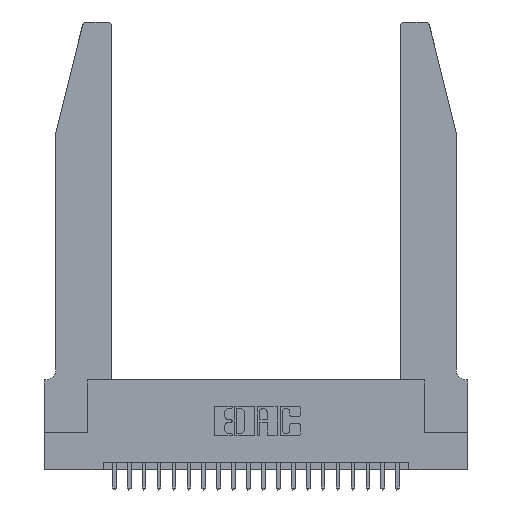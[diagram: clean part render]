
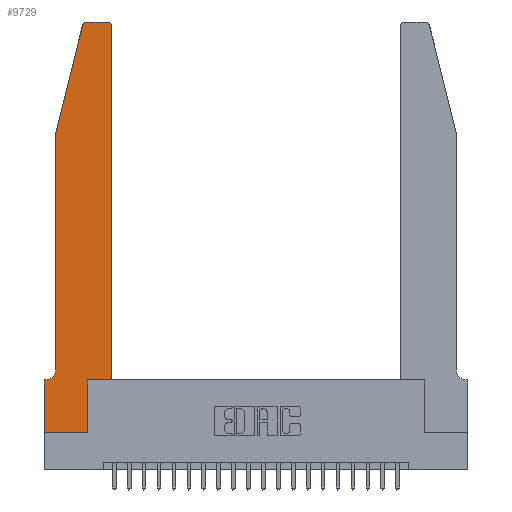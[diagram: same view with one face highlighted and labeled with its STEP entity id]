
A CAD part, top view. The second image highlights one B-rep face of the part: STEP entity #9729.
In plain terms, the highlighted planar face has unit normal (0, 0, 1).
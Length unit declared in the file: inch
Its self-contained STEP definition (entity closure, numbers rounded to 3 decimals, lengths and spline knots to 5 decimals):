
#50 = VERTEX_POINT ( 'NONE', #1312 ) ;
#100 = EDGE_CURVE ( 'NONE', #1104, #11683, #19995, .T. ) ;
#358 = CARTESIAN_POINT ( 'NONE',  ( 0., 0.35, 0.37 ) ) ;
#713 = ORIENTED_EDGE ( 'NONE', *, *, #4176, .T. ) ;
#1104 = VERTEX_POINT ( 'NONE', #2642 ) ;
#1312 = CARTESIAN_POINT ( 'NONE',  ( 0., 0., 0.37 ) ) ;
#1617 = AXIS2_PLACEMENT_3D ( 'NONE', #2029, #14850, #3961 ) ;
#1865 = EDGE_CURVE ( 'NONE', #11683, #8949, #22232, .T. ) ;
#2029 = CARTESIAN_POINT ( 'NONE',  ( 0.284, 2.72, 0.37 ) ) ;
#2412 = DIRECTION ( 'NONE',  ( 0., 1., 0. ) ) ;
#2642 = CARTESIAN_POINT ( 'NONE',  ( 0.0755, 0.42, 0.37 ) ) ;
#2882 = LINE ( 'NONE', #16490, #21459 ) ;
#3354 = ORIENTED_EDGE ( 'NONE', *, *, #100, .T. ) ;
#3527 = DIRECTION ( 'NONE',  ( 0., 1., 0. ) ) ;
#3822 = DIRECTION ( 'NONE',  ( 0., -1., 0. ) ) ;
#3842 = EDGE_CURVE ( 'NONE', #8949, #50, #14447, .T. ) ;
#3961 = DIRECTION ( 'NONE',  ( 1., 0., 0. ) ) ;
#4151 = CARTESIAN_POINT ( 'NONE',  ( 0.4205, 2.72, 0.37 ) ) ;
#4176 = EDGE_CURVE ( 'NONE', #21349, #20176, #12487, .T. ) ;
#4225 = DIRECTION ( 'NONE',  ( 1., 0., 0. ) ) ;
#5479 = ORIENTED_EDGE ( 'NONE', *, *, #12581, .T. ) ;
#5797 = VECTOR ( 'NONE', #16043, 39.37008 ) ;
#6002 = CARTESIAN_POINT ( 'NONE',  ( 0.0755, 2., 0.37 ) ) ;
#6011 = DIRECTION ( 'NONE',  ( 1., 0., 0. ) ) ;
#6042 = ORIENTED_EDGE ( 'NONE', *, *, #21414, .T. ) ;
#6374 = CARTESIAN_POINT ( 'NONE',  ( 0.284, 2.75, 0.37 ) ) ;
#6817 = ORIENTED_EDGE ( 'NONE', *, *, #1865, .T. ) ;
#7343 = CARTESIAN_POINT ( 'NONE',  ( 0.0755, 0.35, 0.37 ) ) ;
#7405 = EDGE_CURVE ( 'NONE', #20176, #19787, #10706, .T. ) ;
#7552 = AXIS2_PLACEMENT_3D ( 'NONE', #4151, #16798, #6011 ) ;
#7586 = EDGE_CURVE ( 'NONE', #13599, #1104, #2882, .T. ) ;
#8742 = EDGE_CURVE ( 'NONE', #14431, #20813, #18527, .T. ) ;
#8949 = VERTEX_POINT ( 'NONE', #10994 ) ;
#9223 = CARTESIAN_POINT ( 'NONE',  ( 0., 0., 0.37 ) ) ;
#9368 = VECTOR ( 'NONE', #3527, 39.37008 ) ;
#9386 = CARTESIAN_POINT ( 'NONE',  ( 0.2865, 0., 0.37 ) ) ;
#9579 = ORIENTED_EDGE ( 'NONE', *, *, #8742, .T. ) ;
#9729 = ADVANCED_FACE ( 'NONE', ( #18483 ), #22086, .T. ) ;
#9760 = AXIS2_PLACEMENT_3D ( 'NONE', #358, #15098, #4225 ) ;
#10150 = VERTEX_POINT ( 'NONE', #17255 ) ;
#10191 = DIRECTION ( 'NONE',  ( 1., 0., 0. ) ) ;
#10476 = LINE ( 'NONE', #11604, #14646 ) ;
#10623 = ORIENTED_EDGE ( 'NONE', *, *, #7405, .T. ) ;
#10706 = LINE ( 'NONE', #21270, #5797 ) ;
#10994 = CARTESIAN_POINT ( 'NONE',  ( 0., 0.35, 0.37 ) ) ;
#11031 = CARTESIAN_POINT ( 'NONE',  ( 0.4505, 0.35, 0.37 ) ) ;
#11354 = AXIS2_PLACEMENT_3D ( 'NONE', #11965, #11962, #11944 ) ;
#11604 = CARTESIAN_POINT ( 'NONE',  ( 0.2865, 0.35, 0.37 ) ) ;
#11683 = VERTEX_POINT ( 'NONE', #14949 ) ;
#11812 = EDGE_LOOP ( 'NONE', ( #10623, #22429, #20871, #18761, #3354, #6817, #16047, #5479, #6042, #9579, #12401, #713 ) ) ;
#11944 = DIRECTION ( 'NONE',  ( -1., 0., 0. ) ) ;
#11947 = VECTOR ( 'NONE', #21605, 39.37008 ) ;
#11962 = DIRECTION ( 'NONE',  ( 0., 0., -1. ) ) ;
#11965 = CARTESIAN_POINT ( 'NONE',  ( 0.0055, 0.42, 0.37 ) ) ;
#12339 = CARTESIAN_POINT ( 'NONE',  ( 0.4505, 0.35, 0.37 ) ) ;
#12401 = ORIENTED_EDGE ( 'NONE', *, *, #14427, .T. ) ;
#12487 = CIRCLE ( 'NONE', #7552, 0.03 ) ;
#12581 = EDGE_CURVE ( 'NONE', #50, #20877, #17802, .T. ) ;
#12828 = VECTOR ( 'NONE', #13495, 39.37008 ) ;
#13127 = VECTOR ( 'NONE', #10191, 39.37008 ) ;
#13495 = DIRECTION ( 'NONE',  ( -0.239, -0.971, 0. ) ) ;
#13599 = VERTEX_POINT ( 'NONE', #6002 ) ;
#13865 = VECTOR ( 'NONE', #21222, 39.37008 ) ;
#14427 = EDGE_CURVE ( 'NONE', #20813, #21349, #22910, .T. ) ;
#14431 = VERTEX_POINT ( 'NONE', #19788 ) ;
#14447 = LINE ( 'NONE', #9223, #11947 ) ;
#14646 = VECTOR ( 'NONE', #2412, 39.37008 ) ;
#14850 = DIRECTION ( 'NONE',  ( 0., 0., 1. ) ) ;
#14949 = CARTESIAN_POINT ( 'NONE',  ( 0.0055, 0.35, 0.37 ) ) ;
#15098 = DIRECTION ( 'NONE',  ( 0., 0., 1. ) ) ;
#15832 = EDGE_CURVE ( 'NONE', #10150, #13599, #22728, .T. ) ;
#16043 = DIRECTION ( 'NONE',  ( -1., 0., 0. ) ) ;
#16047 = ORIENTED_EDGE ( 'NONE', *, *, #3842, .T. ) ;
#16490 = CARTESIAN_POINT ( 'NONE',  ( 0.0755, 2., 0.37 ) ) ;
#16731 = CARTESIAN_POINT ( 'NONE',  ( 0.4505, 2.72, 0.37 ) ) ;
#16798 = DIRECTION ( 'NONE',  ( 0., 0., 1. ) ) ;
#17255 = CARTESIAN_POINT ( 'NONE',  ( 0.25487, 2.72718, 0.37 ) ) ;
#17802 = LINE ( 'NONE', #19028, #13127 ) ;
#17990 = CARTESIAN_POINT ( 'NONE',  ( 0.4505, 0.35, 0.37 ) ) ;
#18123 = VECTOR ( 'NONE', #21614, 39.37008 ) ;
#18483 = FACE_OUTER_BOUND ( 'NONE', #11812, .T. ) ;
#18527 = LINE ( 'NONE', #12339, #13865 ) ;
#18761 = ORIENTED_EDGE ( 'NONE', *, *, #7586, .T. ) ;
#19028 = CARTESIAN_POINT ( 'NONE',  ( 0., 0., 0.37 ) ) ;
#19787 = VERTEX_POINT ( 'NONE', #6374 ) ;
#19788 = CARTESIAN_POINT ( 'NONE',  ( 0.2865, 0.35, 0.37 ) ) ;
#19995 = CIRCLE ( 'NONE', #11354, 0.07 ) ;
#20073 = CARTESIAN_POINT ( 'NONE',  ( 0.4205, 2.75, 0.37 ) ) ;
#20176 = VERTEX_POINT ( 'NONE', #20073 ) ;
#20813 = VERTEX_POINT ( 'NONE', #11031 ) ;
#20871 = ORIENTED_EDGE ( 'NONE', *, *, #15832, .T. ) ;
#20877 = VERTEX_POINT ( 'NONE', #9386 ) ;
#21222 = DIRECTION ( 'NONE',  ( 1., 0., 0. ) ) ;
#21270 = CARTESIAN_POINT ( 'NONE',  ( 0.2605, 2.75, 0.37 ) ) ;
#21349 = VERTEX_POINT ( 'NONE', #16731 ) ;
#21414 = EDGE_CURVE ( 'NONE', #20877, #14431, #10476, .T. ) ;
#21459 = VECTOR ( 'NONE', #3822, 39.37008 ) ;
#21605 = DIRECTION ( 'NONE',  ( 0., -1., 0. ) ) ;
#21614 = DIRECTION ( 'NONE',  ( -1., 0., 0. ) ) ;
#21759 = CIRCLE ( 'NONE', #1617, 0.03 ) ;
#21974 = EDGE_CURVE ( 'NONE', #19787, #10150, #21759, .T. ) ;
#22086 = PLANE ( 'NONE',  #9760 ) ;
#22232 = LINE ( 'NONE', #7343, #18123 ) ;
#22238 = CARTESIAN_POINT ( 'NONE',  ( 0.0755, 2., 0.37 ) ) ;
#22429 = ORIENTED_EDGE ( 'NONE', *, *, #21974, .T. ) ;
#22728 = LINE ( 'NONE', #22238, #12828 ) ;
#22910 = LINE ( 'NONE', #17990, #9368 ) ;
